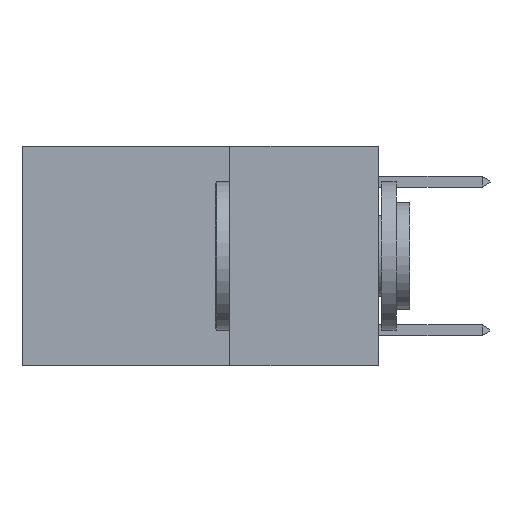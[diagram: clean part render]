
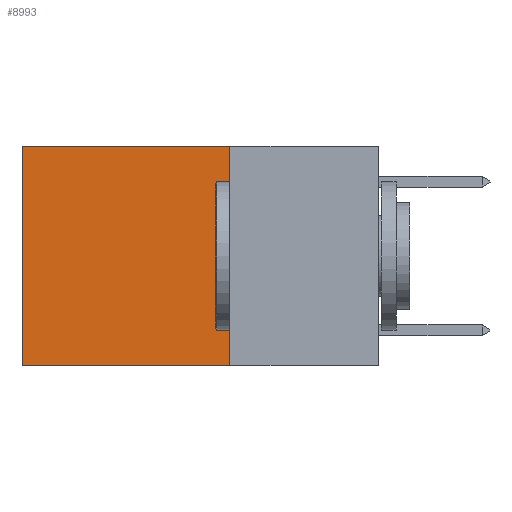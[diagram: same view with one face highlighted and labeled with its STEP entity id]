
A CAD part, left-side view. The second image highlights one B-rep face of the part: STEP entity #8993.
In plain terms, the highlighted planar face has unit normal (-1, 0, 0).
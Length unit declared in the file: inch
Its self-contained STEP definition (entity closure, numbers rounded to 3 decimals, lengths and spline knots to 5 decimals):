
#28 = LINE ( 'NONE', #13213, #11553 ) ;
#70 = VERTEX_POINT ( 'NONE', #7306 ) ;
#222 = EDGE_CURVE ( 'NONE', #13577, #70, #5648, .T. ) ;
#471 = PLANE ( 'NONE',  #10223 ) ;
#662 = VECTOR ( 'NONE', #4747, 39.37008 ) ;
#1887 = EDGE_CURVE ( 'NONE', #70, #7803, #2788, .T. ) ;
#2457 = CARTESIAN_POINT ( 'NONE',  ( 0.2625, 0.25, 0. ) ) ;
#2788 = LINE ( 'NONE', #6108, #5772 ) ;
#2854 = DIRECTION ( 'NONE',  ( 0., 0., -1. ) ) ;
#2917 = DIRECTION ( 'NONE',  ( 0., 1., 0. ) ) ;
#3130 = ORIENTED_EDGE ( 'NONE', *, *, #12782, .F. ) ;
#3663 = ORIENTED_EDGE ( 'NONE', *, *, #1887, .T. ) ;
#3793 = LINE ( 'NONE', #2457, #662 ) ;
#3888 = CARTESIAN_POINT ( 'NONE',  ( 0.2625, 0.25, -0.37 ) ) ;
#4456 = DIRECTION ( 'NONE',  ( 0., 1., 0. ) ) ;
#4747 = DIRECTION ( 'NONE',  ( 0., 0., -1. ) ) ;
#5177 = EDGE_CURVE ( 'NONE', #6093, #7803, #28, .T. ) ;
#5489 = ORIENTED_EDGE ( 'NONE', *, *, #222, .T. ) ;
#5590 = EDGE_LOOP ( 'NONE', ( #3663, #7705, #3130, #5489 ) ) ;
#5648 = LINE ( 'NONE', #10407, #11094 ) ;
#5772 = VECTOR ( 'NONE', #6652, 39.37008 ) ;
#6093 = VERTEX_POINT ( 'NONE', #3888 ) ;
#6108 = CARTESIAN_POINT ( 'NONE',  ( 0.2625, 0.6, 0. ) ) ;
#6652 = DIRECTION ( 'NONE',  ( 0., 0., -1. ) ) ;
#7306 = CARTESIAN_POINT ( 'NONE',  ( 0.2625, 0.6, 0. ) ) ;
#7597 = FACE_OUTER_BOUND ( 'NONE', #5590, .T. ) ;
#7705 = ORIENTED_EDGE ( 'NONE', *, *, #5177, .F. ) ;
#7803 = VERTEX_POINT ( 'NONE', #13922 ) ;
#8355 = CARTESIAN_POINT ( 'NONE',  ( 0.2625, 0.25, 0. ) ) ;
#8993 = ADVANCED_FACE ( 'NONE', ( #7597 ), #471, .F. ) ;
#9439 = DIRECTION ( 'NONE',  ( 1., 0., 0. ) ) ;
#10223 = AXIS2_PLACEMENT_3D ( 'NONE', #8355, #9439, #2854 ) ;
#10407 = CARTESIAN_POINT ( 'NONE',  ( 0.2625, 0.25, 0. ) ) ;
#11094 = VECTOR ( 'NONE', #2917, 39.37008 ) ;
#11097 = CARTESIAN_POINT ( 'NONE',  ( 0.2625, 0.25, 0. ) ) ;
#11553 = VECTOR ( 'NONE', #4456, 39.37008 ) ;
#12782 = EDGE_CURVE ( 'NONE', #13577, #6093, #3793, .T. ) ;
#13213 = CARTESIAN_POINT ( 'NONE',  ( 0.2625, 0.25, -0.37 ) ) ;
#13577 = VERTEX_POINT ( 'NONE', #11097 ) ;
#13922 = CARTESIAN_POINT ( 'NONE',  ( 0.2625, 0.6, -0.37 ) ) ;
